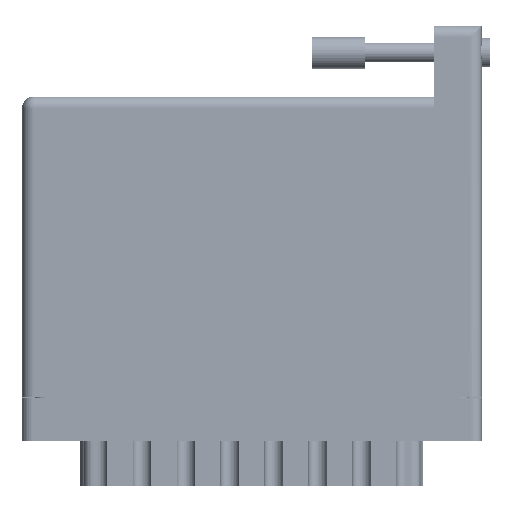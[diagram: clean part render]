
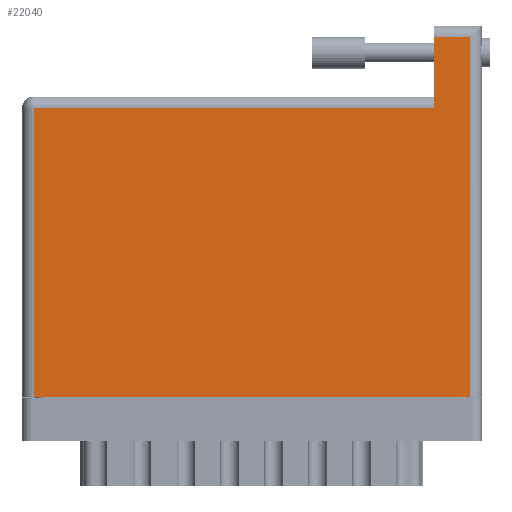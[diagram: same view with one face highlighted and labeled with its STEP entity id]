
A CAD part, front view. The second image highlights one B-rep face of the part: STEP entity #22040.
In plain terms, the highlighted face is planar.
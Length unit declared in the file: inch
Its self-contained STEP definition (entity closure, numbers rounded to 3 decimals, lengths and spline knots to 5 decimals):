
#780 = ORIENTED_EDGE ( 'NONE', *, *, #9656, .T. ) ;
#830 = LINE ( 'NONE', #3870, #31210 ) ;
#1861 = ORIENTED_EDGE ( 'NONE', *, *, #66457, .T. ) ;
#2801 = LINE ( 'NONE', #38757, #33140 ) ;
#3102 = DIRECTION ( 'NONE',  ( 0., 0., -1. ) ) ;
#3870 = CARTESIAN_POINT ( 'NONE',  ( 2.438, 2.195, 0. ) ) ;
#4750 = VERTEX_POINT ( 'NONE', #6978 ) ;
#6978 = CARTESIAN_POINT ( 'NONE',  ( 2.648, 0., 0. ) ) ;
#7979 = EDGE_CURVE ( 'NONE', #58955, #47489, #18909, .T. ) ;
#9656 = EDGE_CURVE ( 'NONE', #4750, #31027, #2801, .T. ) ;
#9697 = VECTOR ( 'NONE', #72298, 39.37008 ) ;
#10204 = ORIENTED_EDGE ( 'NONE', *, *, #50905, .T. ) ;
#13612 = EDGE_CURVE ( 'NONE', #47489, #4750, #18670, .T. ) ;
#18670 = LINE ( 'NONE', #34698, #50116 ) ;
#18909 = LINE ( 'NONE', #71524, #9697 ) ;
#20302 = DIRECTION ( 'NONE',  ( -1., 0., 0. ) ) ;
#22040 = ADVANCED_FACE ( 'NONE', ( #66120 ), #67446, .F. ) ;
#22234 = DIRECTION ( 'NONE',  ( -1., 0., 0. ) ) ;
#26011 = CARTESIAN_POINT ( 'NONE',  ( 0., 1.775, 0. ) ) ;
#27208 = LINE ( 'NONE', #45430, #56749 ) ;
#27871 = CARTESIAN_POINT ( 'NONE',  ( 0.07, 0., 0. ) ) ;
#28286 = ORIENTED_EDGE ( 'NONE', *, *, #7979, .T. ) ;
#29634 = DIRECTION ( 'NONE',  ( -1., 0., 0. ) ) ;
#30833 = AXIS2_PLACEMENT_3D ( 'NONE', #26011, #3102, #20302 ) ;
#31027 = VERTEX_POINT ( 'NONE', #75607 ) ;
#31210 = VECTOR ( 'NONE', #51002, 39.37008 ) ;
#33140 = VECTOR ( 'NONE', #39016, 39.37008 ) ;
#33251 = CARTESIAN_POINT ( 'NONE',  ( 2.438, 2.125, 0. ) ) ;
#34698 = CARTESIAN_POINT ( 'NONE',  ( 0., 0., 0. ) ) ;
#35480 = VERTEX_POINT ( 'NONE', #33251 ) ;
#35847 = EDGE_CURVE ( 'NONE', #48107, #58955, #62463, .T. ) ;
#38757 = CARTESIAN_POINT ( 'NONE',  ( 2.648, 2.195, 0. ) ) ;
#39016 = DIRECTION ( 'NONE',  ( 0., 1., 0. ) ) ;
#40096 = EDGE_LOOP ( 'NONE', ( #41798, #28286, #63761, #780, #10204, #1861 ) ) ;
#41798 = ORIENTED_EDGE ( 'NONE', *, *, #35847, .T. ) ;
#44515 = CARTESIAN_POINT ( 'NONE',  ( 2.438, 1.705, 0. ) ) ;
#45430 = CARTESIAN_POINT ( 'NONE',  ( 0., 2.125, 0. ) ) ;
#45818 = VECTOR ( 'NONE', #29634, 39.37008 ) ;
#46794 = DIRECTION ( 'NONE',  ( 1., 0., 0. ) ) ;
#47489 = VERTEX_POINT ( 'NONE', #27871 ) ;
#48107 = VERTEX_POINT ( 'NONE', #44515 ) ;
#50116 = VECTOR ( 'NONE', #46794, 39.37008 ) ;
#50905 = EDGE_CURVE ( 'NONE', #31027, #35480, #27208, .T. ) ;
#51002 = DIRECTION ( 'NONE',  ( 0., -1., 0. ) ) ;
#56749 = VECTOR ( 'NONE', #22234, 39.37008 ) ;
#58955 = VERTEX_POINT ( 'NONE', #69814 ) ;
#59029 = CARTESIAN_POINT ( 'NONE',  ( 0., 1.705, 0. ) ) ;
#62463 = LINE ( 'NONE', #59029, #45818 ) ;
#63761 = ORIENTED_EDGE ( 'NONE', *, *, #13612, .T. ) ;
#66120 = FACE_OUTER_BOUND ( 'NONE', #40096, .T. ) ;
#66457 = EDGE_CURVE ( 'NONE', #35480, #48107, #830, .T. ) ;
#67446 = PLANE ( 'NONE',  #30833 ) ;
#69814 = CARTESIAN_POINT ( 'NONE',  ( 0.07, 1.705, 0. ) ) ;
#71524 = CARTESIAN_POINT ( 'NONE',  ( 0.07, 0., 0. ) ) ;
#72298 = DIRECTION ( 'NONE',  ( 0., -1., 0. ) ) ;
#75607 = CARTESIAN_POINT ( 'NONE',  ( 2.648, 2.125, 0. ) ) ;
